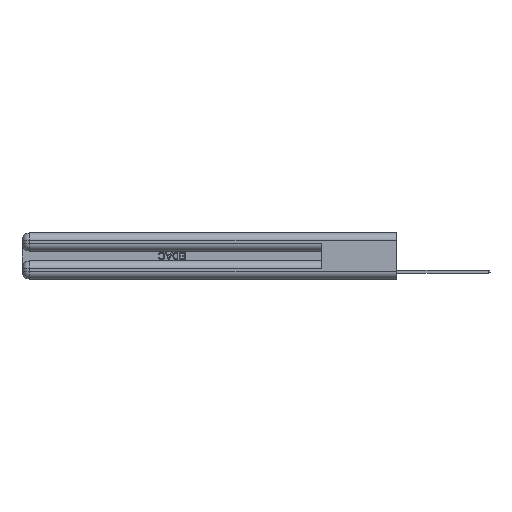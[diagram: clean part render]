
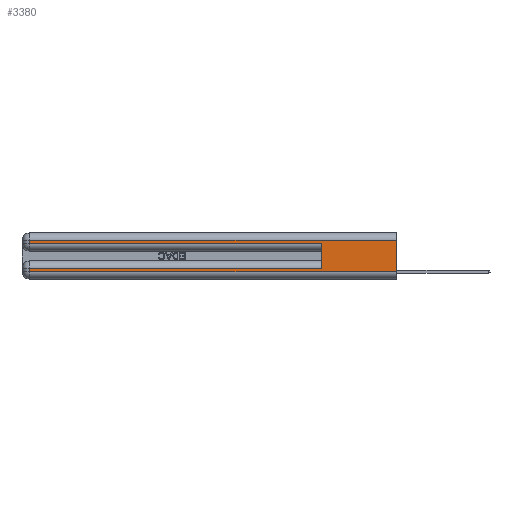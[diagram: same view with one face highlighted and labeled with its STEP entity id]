
A CAD part, left-side view. The second image highlights one B-rep face of the part: STEP entity #3380.
In plain terms, the highlighted planar face has unit normal (-1, 0, 0).
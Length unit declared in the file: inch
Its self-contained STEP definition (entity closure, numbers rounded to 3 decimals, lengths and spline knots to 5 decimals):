
#28 = VERTEX_POINT ( 'NONE', #11002 ) ;
#432 = CARTESIAN_POINT ( 'NONE',  ( 0., 0.6, 0.085 ) ) ;
#1229 = LINE ( 'NONE', #1428, #30369 ) ;
#1243 = CARTESIAN_POINT ( 'NONE',  ( 0., 0.6, 0.285 ) ) ;
#1428 = CARTESIAN_POINT ( 'NONE',  ( 0., 0., 0.06 ) ) ;
#1760 = DIRECTION ( 'NONE',  ( 0., 0., -1. ) ) ;
#2072 = EDGE_CURVE ( 'NONE', #2556, #9284, #29201, .T. ) ;
#2077 = CARTESIAN_POINT ( 'NONE',  ( 0., 2.94, 0.085 ) ) ;
#2556 = VERTEX_POINT ( 'NONE', #432 ) ;
#3170 = VECTOR ( 'NONE', #22315, 39.37008 ) ;
#3380 = ADVANCED_FACE ( 'NONE', ( #23738 ), #15966, .F. ) ;
#4319 = DIRECTION ( 'NONE',  ( 0., -1., 0. ) ) ;
#4469 = VECTOR ( 'NONE', #1760, 39.37008 ) ;
#4793 = EDGE_CURVE ( 'NONE', #10799, #22889, #14760, .T. ) ;
#5339 = CARTESIAN_POINT ( 'NONE',  ( 0., 2.94, 0.37 ) ) ;
#5814 = LINE ( 'NONE', #5339, #3170 ) ;
#7043 = DIRECTION ( 'NONE',  ( 0., 0., -1. ) ) ;
#7359 = DIRECTION ( 'NONE',  ( 0., 1., 0. ) ) ;
#8520 = CARTESIAN_POINT ( 'NONE',  ( 0., 2.94, 0.31 ) ) ;
#8645 = VECTOR ( 'NONE', #7043, 39.37008 ) ;
#8936 = CARTESIAN_POINT ( 'NONE',  ( 0., 2.94, 0.37 ) ) ;
#9284 = VERTEX_POINT ( 'NONE', #1243 ) ;
#9743 = DIRECTION ( 'NONE',  ( 0., 1., 0. ) ) ;
#10517 = EDGE_CURVE ( 'NONE', #2556, #28772, #29113, .T. ) ;
#10576 = ORIENTED_EDGE ( 'NONE', *, *, #10517, .T. ) ;
#10799 = VERTEX_POINT ( 'NONE', #8520 ) ;
#11002 = CARTESIAN_POINT ( 'NONE',  ( 0., 2.94, 0.06 ) ) ;
#11401 = DIRECTION ( 'NONE',  ( 1., 0., 0. ) ) ;
#11642 = CARTESIAN_POINT ( 'NONE',  ( 0., 0., 0.31 ) ) ;
#11854 = CARTESIAN_POINT ( 'NONE',  ( 0., 0., 0.37 ) ) ;
#13407 = VECTOR ( 'NONE', #7359, 39.37008 ) ;
#14259 = CARTESIAN_POINT ( 'NONE',  ( 0., 0., 0.31 ) ) ;
#14760 = LINE ( 'NONE', #8936, #4469 ) ;
#15080 = ORIENTED_EDGE ( 'NONE', *, *, #19609, .F. ) ;
#15942 = ORIENTED_EDGE ( 'NONE', *, *, #4793, .T. ) ;
#15966 = PLANE ( 'NONE',  #28015 ) ;
#16082 = CARTESIAN_POINT ( 'NONE',  ( 0., 0., 0.37 ) ) ;
#16876 = VECTOR ( 'NONE', #30398, 39.37008 ) ;
#16965 = CARTESIAN_POINT ( 'NONE',  ( 0., 0., 0.085 ) ) ;
#17087 = EDGE_CURVE ( 'NONE', #20724, #10799, #22615, .T. ) ;
#17499 = VERTEX_POINT ( 'NONE', #31477 ) ;
#17763 = CARTESIAN_POINT ( 'NONE',  ( 0., 0.6, 0.145 ) ) ;
#18839 = DIRECTION ( 'NONE',  ( 0., 0., -1. ) ) ;
#18869 = ORIENTED_EDGE ( 'NONE', *, *, #30467, .T. ) ;
#19609 = EDGE_CURVE ( 'NONE', #20724, #17499, #31286, .T. ) ;
#20260 = EDGE_CURVE ( 'NONE', #22889, #9284, #25472, .T. ) ;
#20724 = VERTEX_POINT ( 'NONE', #11642 ) ;
#21894 = ORIENTED_EDGE ( 'NONE', *, *, #20260, .T. ) ;
#22315 = DIRECTION ( 'NONE',  ( 0., 0., -1. ) ) ;
#22615 = LINE ( 'NONE', #14259, #13407 ) ;
#22889 = VERTEX_POINT ( 'NONE', #29461 ) ;
#23738 = FACE_OUTER_BOUND ( 'NONE', #30578, .T. ) ;
#24226 = EDGE_CURVE ( 'NONE', #28772, #28, #5814, .T. ) ;
#24445 = ORIENTED_EDGE ( 'NONE', *, *, #24226, .T. ) ;
#24674 = ORIENTED_EDGE ( 'NONE', *, *, #17087, .T. ) ;
#24705 = DIRECTION ( 'NONE',  ( 0., -1., 0. ) ) ;
#24739 = ORIENTED_EDGE ( 'NONE', *, *, #2072, .F. ) ;
#25472 = LINE ( 'NONE', #29771, #28173 ) ;
#26442 = VECTOR ( 'NONE', #9743, 39.37008 ) ;
#28015 = AXIS2_PLACEMENT_3D ( 'NONE', #16082, #11401, #18839 ) ;
#28173 = VECTOR ( 'NONE', #24705, 39.37008 ) ;
#28772 = VERTEX_POINT ( 'NONE', #2077 ) ;
#29113 = LINE ( 'NONE', #16965, #26442 ) ;
#29201 = LINE ( 'NONE', #17763, #16876 ) ;
#29461 = CARTESIAN_POINT ( 'NONE',  ( 0., 2.94, 0.285 ) ) ;
#29771 = CARTESIAN_POINT ( 'NONE',  ( 0., 0., 0.285 ) ) ;
#30369 = VECTOR ( 'NONE', #4319, 39.37008 ) ;
#30398 = DIRECTION ( 'NONE',  ( 0., 0., 1. ) ) ;
#30467 = EDGE_CURVE ( 'NONE', #28, #17499, #1229, .T. ) ;
#30578 = EDGE_LOOP ( 'NONE', ( #15080, #24674, #15942, #21894, #24739, #10576, #24445, #18869 ) ) ;
#31286 = LINE ( 'NONE', #11854, #8645 ) ;
#31477 = CARTESIAN_POINT ( 'NONE',  ( 0., 0., 0.06 ) ) ;
